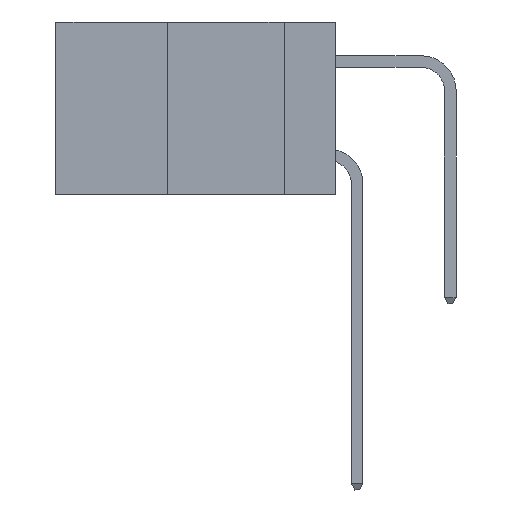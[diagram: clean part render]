
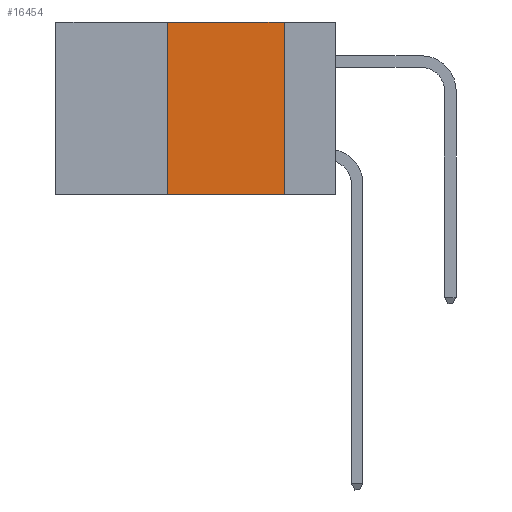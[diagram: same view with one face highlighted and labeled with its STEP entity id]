
A CAD part, left-side view. The second image highlights one B-rep face of the part: STEP entity #16454.
In plain terms, the highlighted planar face has unit normal (-1, 0, 0).
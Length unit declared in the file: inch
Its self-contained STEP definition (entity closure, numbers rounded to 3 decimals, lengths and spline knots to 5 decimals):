
#1759 = VERTEX_POINT ( 'NONE', #19378 ) ;
#1825 = CARTESIAN_POINT ( 'NONE',  ( 0., 0.11, -0.37 ) ) ;
#3274 = VECTOR ( 'NONE', #28715, 39.37008 ) ;
#3436 = CARTESIAN_POINT ( 'NONE',  ( 0., 0.6, -0.37 ) ) ;
#5122 = FACE_OUTER_BOUND ( 'NONE', #23158, .T. ) ;
#5777 = CARTESIAN_POINT ( 'NONE',  ( 0., 0.36, 0. ) ) ;
#6383 = DIRECTION ( 'NONE',  ( 1., 0., 0. ) ) ;
#7261 = AXIS2_PLACEMENT_3D ( 'NONE', #18499, #6383, #41023 ) ;
#7455 = VECTOR ( 'NONE', #40862, 39.37008 ) ;
#8789 = VERTEX_POINT ( 'NONE', #31581 ) ;
#10383 = LINE ( 'NONE', #27510, #26331 ) ;
#11633 = DIRECTION ( 'NONE',  ( 0., 0., -1. ) ) ;
#11774 = LINE ( 'NONE', #38157, #3274 ) ;
#12093 = PLANE ( 'NONE',  #7261 ) ;
#14268 = ORIENTED_EDGE ( 'NONE', *, *, #33538, .F. ) ;
#16454 = ADVANCED_FACE ( 'NONE', ( #5122 ), #12093, .F. ) ;
#16608 = EDGE_CURVE ( 'NONE', #31074, #33842, #29586, .T. ) ;
#18499 = CARTESIAN_POINT ( 'NONE',  ( 0., 0.6, 0. ) ) ;
#19378 = CARTESIAN_POINT ( 'NONE',  ( 0., 0.11, 0. ) ) ;
#21050 = ORIENTED_EDGE ( 'NONE', *, *, #34913, .F. ) ;
#21060 = VECTOR ( 'NONE', #28966, 39.37008 ) ;
#23158 = EDGE_LOOP ( 'NONE', ( #37172, #21050, #14268, #33824 ) ) ;
#26283 = CARTESIAN_POINT ( 'NONE',  ( 0., 0.36, -0.37 ) ) ;
#26331 = VECTOR ( 'NONE', #11633, 39.37008 ) ;
#26822 = EDGE_CURVE ( 'NONE', #1759, #33842, #10383, .T. ) ;
#27510 = CARTESIAN_POINT ( 'NONE',  ( 0., 0.11, 0. ) ) ;
#28715 = DIRECTION ( 'NONE',  ( 0., -1., 0. ) ) ;
#28966 = DIRECTION ( 'NONE',  ( 0., -1., 0. ) ) ;
#29586 = LINE ( 'NONE', #3436, #21060 ) ;
#31074 = VERTEX_POINT ( 'NONE', #26283 ) ;
#31581 = CARTESIAN_POINT ( 'NONE',  ( 0., 0.36, 0. ) ) ;
#33328 = LINE ( 'NONE', #5777, #7455 ) ;
#33538 = EDGE_CURVE ( 'NONE', #31074, #8789, #33328, .T. ) ;
#33824 = ORIENTED_EDGE ( 'NONE', *, *, #16608, .T. ) ;
#33842 = VERTEX_POINT ( 'NONE', #1825 ) ;
#34913 = EDGE_CURVE ( 'NONE', #8789, #1759, #11774, .T. ) ;
#37172 = ORIENTED_EDGE ( 'NONE', *, *, #26822, .F. ) ;
#38157 = CARTESIAN_POINT ( 'NONE',  ( 0., 0.6, 0. ) ) ;
#40862 = DIRECTION ( 'NONE',  ( 0., 0., 1. ) ) ;
#41023 = DIRECTION ( 'NONE',  ( 0., 0., -1. ) ) ;
